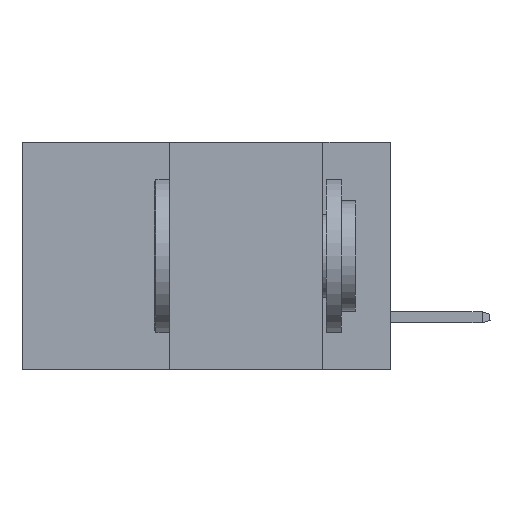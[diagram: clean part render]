
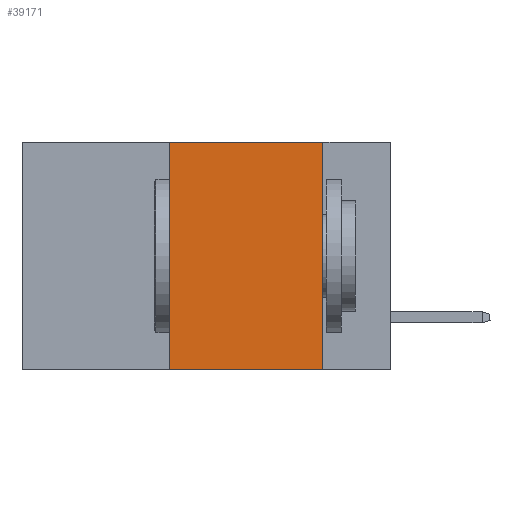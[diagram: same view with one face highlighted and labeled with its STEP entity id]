
A CAD part, left-side view. The second image highlights one B-rep face of the part: STEP entity #39171.
In plain terms, the highlighted planar face has unit normal (-1, 0, 0).
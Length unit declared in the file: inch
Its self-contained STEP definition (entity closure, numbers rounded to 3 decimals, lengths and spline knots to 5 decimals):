
#378 = EDGE_CURVE ( 'NONE', #11295, #33256, #25890, .T. ) ;
#542 = DIRECTION ( 'NONE',  ( 0., 0., -1. ) ) ;
#1309 = EDGE_CURVE ( 'NONE', #11295, #22188, #24865, .T. ) ;
#1470 = CARTESIAN_POINT ( 'NONE',  ( 0., 0.11, 0. ) ) ;
#3210 = DIRECTION ( 'NONE',  ( 0., -1., 0. ) ) ;
#5484 = DIRECTION ( 'NONE',  ( 0., -1., 0. ) ) ;
#5515 = VECTOR ( 'NONE', #5484, 39.37008 ) ;
#6614 = EDGE_CURVE ( 'NONE', #16026, #33256, #13378, .T. ) ;
#8433 = ORIENTED_EDGE ( 'NONE', *, *, #1309, .F. ) ;
#9204 = EDGE_LOOP ( 'NONE', ( #25219, #25958, #8433, #30047 ) ) ;
#10269 = CARTESIAN_POINT ( 'NONE',  ( 0., 0.36, 0. ) ) ;
#11295 = VERTEX_POINT ( 'NONE', #32901 ) ;
#11385 = DIRECTION ( 'NONE',  ( 0., 0., 1. ) ) ;
#11629 = DIRECTION ( 'NONE',  ( 0., 0., -1. ) ) ;
#13378 = LINE ( 'NONE', #24692, #28538 ) ;
#14759 = AXIS2_PLACEMENT_3D ( 'NONE', #17831, #17447, #11629 ) ;
#16026 = VERTEX_POINT ( 'NONE', #1470 ) ;
#17447 = DIRECTION ( 'NONE',  ( 1., 0., 0. ) ) ;
#17831 = CARTESIAN_POINT ( 'NONE',  ( 0., 0.6, 0. ) ) ;
#20551 = EDGE_CURVE ( 'NONE', #22188, #16026, #21331, .T. ) ;
#21331 = LINE ( 'NONE', #39285, #22266 ) ;
#22188 = VERTEX_POINT ( 'NONE', #10269 ) ;
#22266 = VECTOR ( 'NONE', #3210, 39.37008 ) ;
#23456 = VECTOR ( 'NONE', #11385, 39.37008 ) ;
#24692 = CARTESIAN_POINT ( 'NONE',  ( 0., 0.11, 0. ) ) ;
#24858 = CARTESIAN_POINT ( 'NONE',  ( 0., 0.11, -0.37 ) ) ;
#24865 = LINE ( 'NONE', #32409, #23456 ) ;
#25219 = ORIENTED_EDGE ( 'NONE', *, *, #6614, .F. ) ;
#25776 = CARTESIAN_POINT ( 'NONE',  ( 0., 0.6, -0.37 ) ) ;
#25890 = LINE ( 'NONE', #25776, #5515 ) ;
#25958 = ORIENTED_EDGE ( 'NONE', *, *, #20551, .F. ) ;
#26960 = PLANE ( 'NONE',  #14759 ) ;
#28538 = VECTOR ( 'NONE', #542, 39.37008 ) ;
#30047 = ORIENTED_EDGE ( 'NONE', *, *, #378, .T. ) ;
#32409 = CARTESIAN_POINT ( 'NONE',  ( 0., 0.36, 0. ) ) ;
#32901 = CARTESIAN_POINT ( 'NONE',  ( 0., 0.36, -0.37 ) ) ;
#33256 = VERTEX_POINT ( 'NONE', #24858 ) ;
#39157 = FACE_OUTER_BOUND ( 'NONE', #9204, .T. ) ;
#39171 = ADVANCED_FACE ( 'NONE', ( #39157 ), #26960, .F. ) ;
#39285 = CARTESIAN_POINT ( 'NONE',  ( 0., 0.6, 0. ) ) ;
